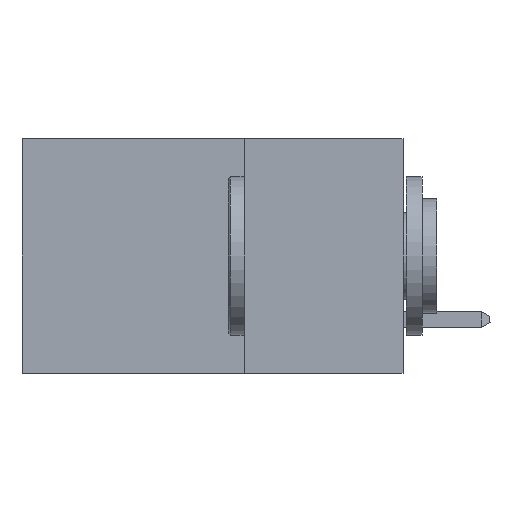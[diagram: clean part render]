
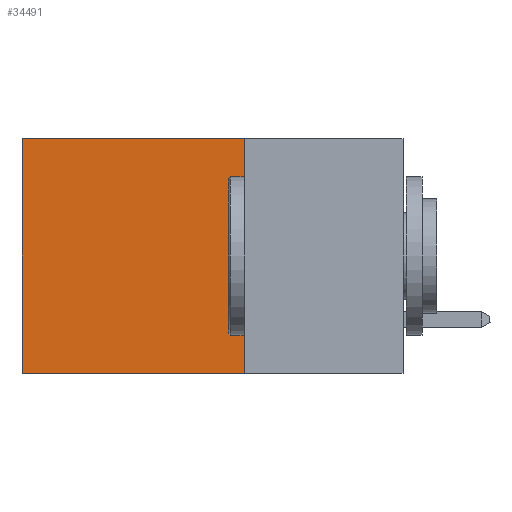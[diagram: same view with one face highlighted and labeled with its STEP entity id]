
A CAD part, left-side view. The second image highlights one B-rep face of the part: STEP entity #34491.
In plain terms, the highlighted planar face has unit normal (-1, 0, 0).
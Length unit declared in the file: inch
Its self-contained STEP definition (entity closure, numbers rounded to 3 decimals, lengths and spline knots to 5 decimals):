
#988 = CARTESIAN_POINT ( 'NONE',  ( 0.2875, 0.6, -0.37 ) ) ;
#3015 = DIRECTION ( 'NONE',  ( 0., 0., -1. ) ) ;
#3067 = DIRECTION ( 'NONE',  ( 0., 1., 0. ) ) ;
#3287 = ORIENTED_EDGE ( 'NONE', *, *, #12837, .T. ) ;
#4968 = VECTOR ( 'NONE', #42082, 39.37008 ) ;
#5217 = AXIS2_PLACEMENT_3D ( 'NONE', #23696, #42825, #30978 ) ;
#6540 = CARTESIAN_POINT ( 'NONE',  ( 0.2875, 0.25, 0. ) ) ;
#7183 = EDGE_LOOP ( 'NONE', ( #3287, #14033, #14113, #7355 ) ) ;
#7355 = ORIENTED_EDGE ( 'NONE', *, *, #31922, .T. ) ;
#8178 = LINE ( 'NONE', #45114, #39038 ) ;
#12837 = EDGE_CURVE ( 'NONE', #18661, #48964, #8178, .T. ) ;
#13101 = VECTOR ( 'NONE', #48826, 39.37008 ) ;
#14033 = ORIENTED_EDGE ( 'NONE', *, *, #37608, .F. ) ;
#14113 = ORIENTED_EDGE ( 'NONE', *, *, #42231, .F. ) ;
#16072 = LINE ( 'NONE', #37579, #49446 ) ;
#18661 = VERTEX_POINT ( 'NONE', #25999 ) ;
#19818 = PLANE ( 'NONE',  #5217 ) ;
#21336 = LINE ( 'NONE', #38221, #4968 ) ;
#22872 = LINE ( 'NONE', #6540, #13101 ) ;
#23696 = CARTESIAN_POINT ( 'NONE',  ( 0.2875, 0.25, 0. ) ) ;
#25999 = CARTESIAN_POINT ( 'NONE',  ( 0.2875, 0.6, 0. ) ) ;
#30978 = DIRECTION ( 'NONE',  ( 0., 0., -1. ) ) ;
#31922 = EDGE_CURVE ( 'NONE', #36394, #18661, #21336, .T. ) ;
#34491 = ADVANCED_FACE ( 'NONE', ( #42294 ), #19818, .F. ) ;
#34671 = CARTESIAN_POINT ( 'NONE',  ( 0.2875, 0.25, 0. ) ) ;
#36394 = VERTEX_POINT ( 'NONE', #34671 ) ;
#37579 = CARTESIAN_POINT ( 'NONE',  ( 0.2875, 0.25, -0.37 ) ) ;
#37608 = EDGE_CURVE ( 'NONE', #47817, #48964, #16072, .T. ) ;
#38221 = CARTESIAN_POINT ( 'NONE',  ( 0.2875, 0.25, 0. ) ) ;
#39038 = VECTOR ( 'NONE', #3015, 39.37008 ) ;
#42082 = DIRECTION ( 'NONE',  ( 0., 1., 0. ) ) ;
#42231 = EDGE_CURVE ( 'NONE', #36394, #47817, #22872, .T. ) ;
#42294 = FACE_OUTER_BOUND ( 'NONE', #7183, .T. ) ;
#42825 = DIRECTION ( 'NONE',  ( 1., 0., 0. ) ) ;
#45114 = CARTESIAN_POINT ( 'NONE',  ( 0.2875, 0.6, 0. ) ) ;
#47817 = VERTEX_POINT ( 'NONE', #48010 ) ;
#48010 = CARTESIAN_POINT ( 'NONE',  ( 0.2875, 0.25, -0.37 ) ) ;
#48826 = DIRECTION ( 'NONE',  ( 0., 0., -1. ) ) ;
#48964 = VERTEX_POINT ( 'NONE', #988 ) ;
#49446 = VECTOR ( 'NONE', #3067, 39.37008 ) ;
